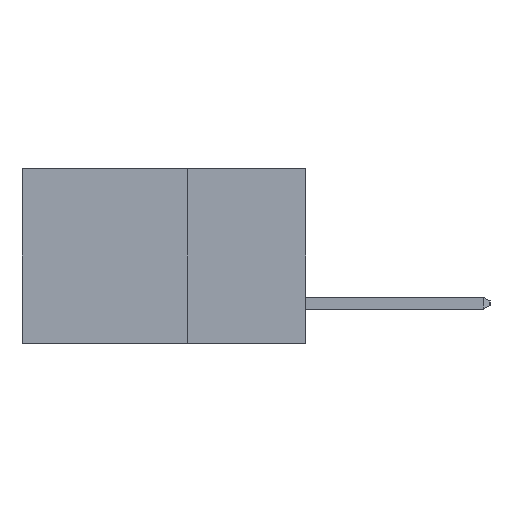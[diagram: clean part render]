
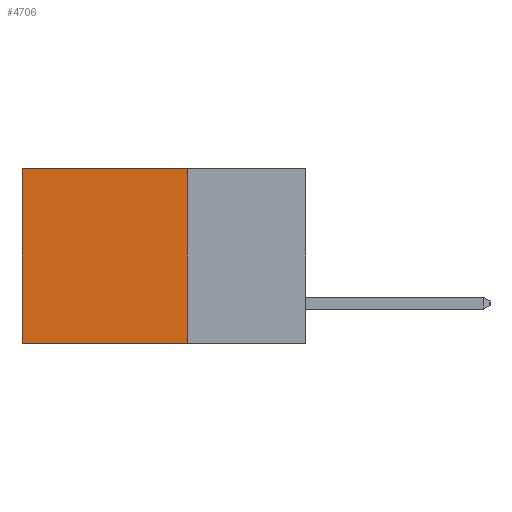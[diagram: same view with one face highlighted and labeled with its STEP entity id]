
A CAD part, left-side view. The second image highlights one B-rep face of the part: STEP entity #4706.
In plain terms, the highlighted planar face has unit normal (-1, 0, 0).
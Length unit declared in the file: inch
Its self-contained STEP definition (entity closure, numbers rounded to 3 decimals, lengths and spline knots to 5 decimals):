
#518 = VERTEX_POINT ( 'NONE', #16554 ) ;
#846 = VECTOR ( 'NONE', #21943, 39.37008 ) ;
#1437 = LINE ( 'NONE', #6455, #846 ) ;
#2795 = CARTESIAN_POINT ( 'NONE',  ( 0.298, 0.25, 0. ) ) ;
#3024 = ORIENTED_EDGE ( 'NONE', *, *, #4025, .T. ) ;
#3404 = CARTESIAN_POINT ( 'NONE',  ( 0.298, 0.25, -0.37 ) ) ;
#4025 = EDGE_CURVE ( 'NONE', #19722, #518, #5782, .T. ) ;
#4362 = CARTESIAN_POINT ( 'NONE',  ( 0.298, 0.6, 0. ) ) ;
#4706 = ADVANCED_FACE ( 'NONE', ( #5491 ), #9976, .F. ) ;
#5096 = ORIENTED_EDGE ( 'NONE', *, *, #21501, .F. ) ;
#5491 = FACE_OUTER_BOUND ( 'NONE', #15785, .T. ) ;
#5782 = LINE ( 'NONE', #16030, #14521 ) ;
#5859 = VERTEX_POINT ( 'NONE', #3404 ) ;
#6161 = DIRECTION ( 'NONE',  ( 0., 0., -1. ) ) ;
#6455 = CARTESIAN_POINT ( 'NONE',  ( 0.298, 0.25, -0.37 ) ) ;
#6887 = AXIS2_PLACEMENT_3D ( 'NONE', #9922, #10313, #10287 ) ;
#7274 = LINE ( 'NONE', #4362, #15994 ) ;
#7586 = ORIENTED_EDGE ( 'NONE', *, *, #22295, .F. ) ;
#9523 = VERTEX_POINT ( 'NONE', #14564 ) ;
#9922 = CARTESIAN_POINT ( 'NONE',  ( 0.298, 0.25, 0. ) ) ;
#9976 = PLANE ( 'NONE',  #6887 ) ;
#10287 = DIRECTION ( 'NONE',  ( 0., 0., -1. ) ) ;
#10313 = DIRECTION ( 'NONE',  ( 1., 0., 0. ) ) ;
#11208 = VECTOR ( 'NONE', #20932, 39.37008 ) ;
#13691 = EDGE_CURVE ( 'NONE', #518, #9523, #7274, .T. ) ;
#14521 = VECTOR ( 'NONE', #15896, 39.37008 ) ;
#14564 = CARTESIAN_POINT ( 'NONE',  ( 0.298, 0.6, -0.37 ) ) ;
#15785 = EDGE_LOOP ( 'NONE', ( #20855, #5096, #7586, #3024 ) ) ;
#15896 = DIRECTION ( 'NONE',  ( 0., 1., 0. ) ) ;
#15994 = VECTOR ( 'NONE', #6161, 39.37008 ) ;
#16030 = CARTESIAN_POINT ( 'NONE',  ( 0.298, 0.25, 0. ) ) ;
#16554 = CARTESIAN_POINT ( 'NONE',  ( 0.298, 0.6, 0. ) ) ;
#19230 = CARTESIAN_POINT ( 'NONE',  ( 0.298, 0.25, 0. ) ) ;
#19722 = VERTEX_POINT ( 'NONE', #2795 ) ;
#20340 = LINE ( 'NONE', #19230, #11208 ) ;
#20855 = ORIENTED_EDGE ( 'NONE', *, *, #13691, .T. ) ;
#20932 = DIRECTION ( 'NONE',  ( 0., 0., -1. ) ) ;
#21501 = EDGE_CURVE ( 'NONE', #5859, #9523, #1437, .T. ) ;
#21943 = DIRECTION ( 'NONE',  ( 0., 1., 0. ) ) ;
#22295 = EDGE_CURVE ( 'NONE', #19722, #5859, #20340, .T. ) ;
